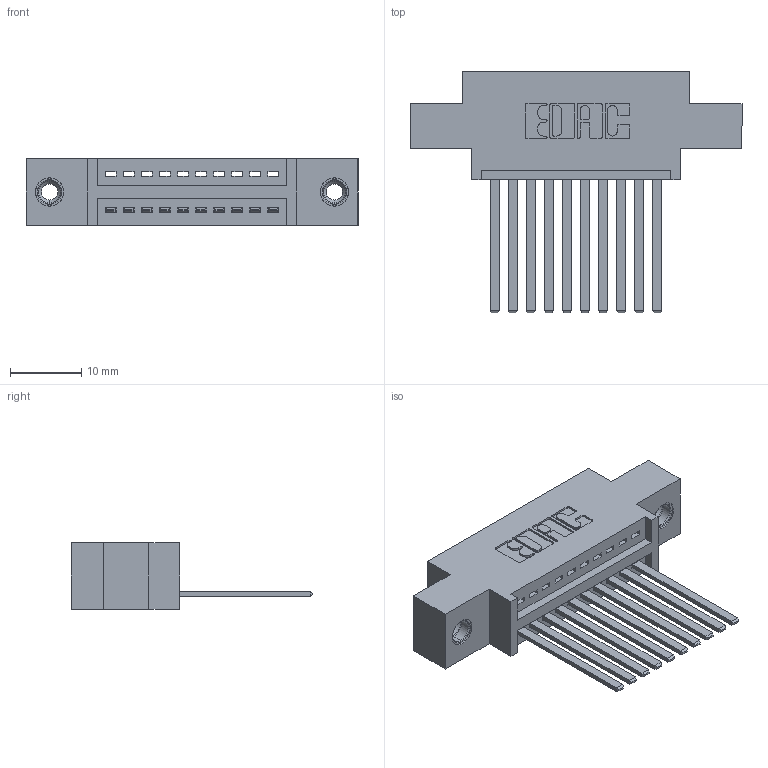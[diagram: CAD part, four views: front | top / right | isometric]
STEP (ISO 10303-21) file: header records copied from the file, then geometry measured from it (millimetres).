
FILE_DESCRIPTION (( 'STEP AP203' ), '1' );
FILE_NAME ('395-010-544-608.STEP', '2018-11-02T14:07:57', ( '' ), ( '' ), 'SwSTEP 2.0', 'SolidWorks 2016', '' );
FILE_SCHEMA (( 'CONFIG_CONTROL_DESIGN' ));
Length unit declared in the file: inch
Products named in the file (4): 395-010-544-608; 345-292-001_345-293-144; 345-250-001_345-250-003-102; 345 Part_0.170 Offset - 0.156 Dia-TI
Assembly tree (13 placements, depth 2):
  395-010-544-608
    345 Part_0.170 Offset - 0.156 Dia-TI
    345-292-001_345-293-144  x10
    345-250-001_345-250-003-102  x2
Bounding box: 46.61 x 33.96 x 9.4 mm (x, y, z)
Volume: 4160.8 mm3; surface area: 5587.7 mm2
Topology: 13 solids, 13 shells, 710 faces, 2069 edges, 1358 vertices
Faces by surface type: plane 476, cylinder 218, cone 12, torus 4
Entity records: 12968 total; most frequent: CARTESIAN_POINT 2229, ORIENTED_EDGE 2166, DIRECTION 2017, EDGE_CURVE 1083, VECTOR 895, LINE 895, VERTEX_POINT 716, AXIS2_PLACEMENT_3D 561
